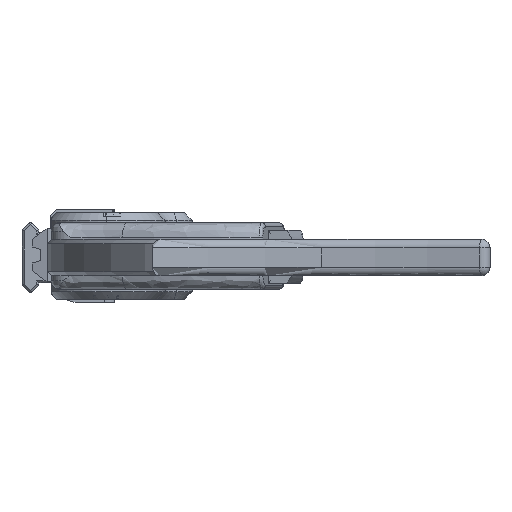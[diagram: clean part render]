
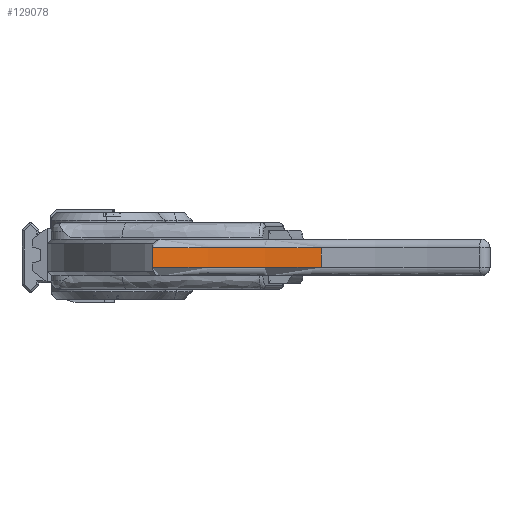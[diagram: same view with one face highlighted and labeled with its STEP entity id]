
A CAD part, left-side view. The second image highlights one B-rep face of the part: STEP entity #129078.
In plain terms, the highlighted cylindrical face has radius 203.2 mm (diameter 406.4 mm), a partial arc.
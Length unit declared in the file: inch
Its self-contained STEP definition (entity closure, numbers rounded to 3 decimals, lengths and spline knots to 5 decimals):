
#3450 = CARTESIAN_POINT ( 'NONE',  ( -15.87043, -1.16875, -15.38501 ) ) ;
#5020 = AXIS2_PLACEMENT_3D ( 'NONE', #93368, #92628, #210418 ) ;
#21212 = DIRECTION ( 'NONE',  ( 0., 0., 1. ) ) ;
#34251 = CIRCLE ( 'NONE', #5020, 8. ) ;
#42677 = CARTESIAN_POINT ( 'NONE',  ( -23.87043, -1.16875, -0.1 ) ) ;
#56366 = ORIENTED_EDGE ( 'NONE', *, *, #177128, .T. ) ;
#68883 = AXIS2_PLACEMENT_3D ( 'NONE', #153858, #151627, #158204 ) ;
#74726 = CARTESIAN_POINT ( 'NONE',  ( -16.12446, 0.83125, -0.333 ) ) ;
#81566 = LINE ( 'NONE', #3450, #179730 ) ;
#82500 = AXIS2_PLACEMENT_3D ( 'NONE', #42677, #94597, #112409 ) ;
#84360 = CARTESIAN_POINT ( 'NONE',  ( -16.12446, 0.83125, -0.1 ) ) ;
#85142 = ORIENTED_EDGE ( 'NONE', *, *, #152520, .T. ) ;
#90139 = LINE ( 'NONE', #99893, #119341 ) ;
#90505 = FACE_OUTER_BOUND ( 'NONE', #127126, .T. ) ;
#92628 = DIRECTION ( 'NONE',  ( 0., 0., -1. ) ) ;
#93368 = CARTESIAN_POINT ( 'NONE',  ( -23.87043, -1.16875, -0.333 ) ) ;
#94597 = DIRECTION ( 'NONE',  ( 0., 0., 1. ) ) ;
#95320 = VERTEX_POINT ( 'NONE', #84360 ) ;
#99893 = CARTESIAN_POINT ( 'NONE',  ( -16.12446, 0.83125, -15.38501 ) ) ;
#109052 = CYLINDRICAL_SURFACE ( 'NONE', #68883, 8. ) ;
#112409 = DIRECTION ( 'NONE',  ( -1., 0., 0. ) ) ;
#118635 = CIRCLE ( 'NONE', #82500, 8. ) ;
#119341 = VECTOR ( 'NONE', #134734, 39.37008 ) ;
#127126 = EDGE_LOOP ( 'NONE', ( #56366, #135292, #85142, #149171 ) ) ;
#129078 = ADVANCED_FACE ( 'NONE', ( #90505 ), #109052, .F. ) ;
#132161 = VERTEX_POINT ( 'NONE', #74726 ) ;
#134734 = DIRECTION ( 'NONE',  ( 0., 0., 1. ) ) ;
#135292 = ORIENTED_EDGE ( 'NONE', *, *, #211923, .T. ) ;
#146757 = CARTESIAN_POINT ( 'NONE',  ( -15.87043, -1.16875, -0.1 ) ) ;
#149171 = ORIENTED_EDGE ( 'NONE', *, *, #187328, .F. ) ;
#151627 = DIRECTION ( 'NONE',  ( 0., 0., 1. ) ) ;
#152520 = EDGE_CURVE ( 'NONE', #200520, #95320, #118635, .T. ) ;
#153858 = CARTESIAN_POINT ( 'NONE',  ( -23.87043, -1.16875, -15.38501 ) ) ;
#155312 = CARTESIAN_POINT ( 'NONE',  ( -15.87043, -1.16875, -0.333 ) ) ;
#158204 = DIRECTION ( 'NONE',  ( 1., 0., 0. ) ) ;
#175797 = VERTEX_POINT ( 'NONE', #155312 ) ;
#177128 = EDGE_CURVE ( 'NONE', #132161, #175797, #34251, .T. ) ;
#179730 = VECTOR ( 'NONE', #21212, 39.37008 ) ;
#187328 = EDGE_CURVE ( 'NONE', #132161, #95320, #90139, .T. ) ;
#200520 = VERTEX_POINT ( 'NONE', #146757 ) ;
#210418 = DIRECTION ( 'NONE',  ( -1., 0., 0. ) ) ;
#211923 = EDGE_CURVE ( 'NONE', #175797, #200520, #81566, .T. ) ;
